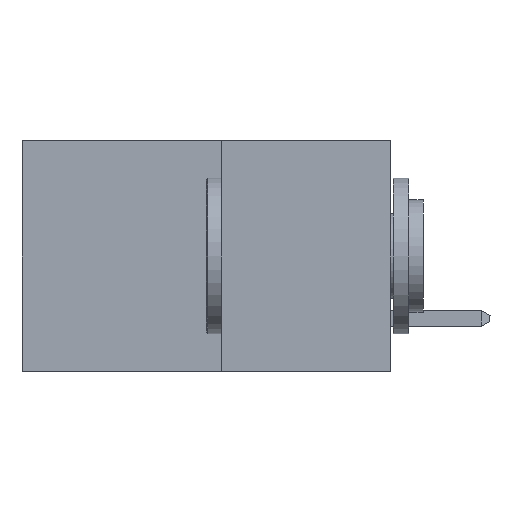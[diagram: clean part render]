
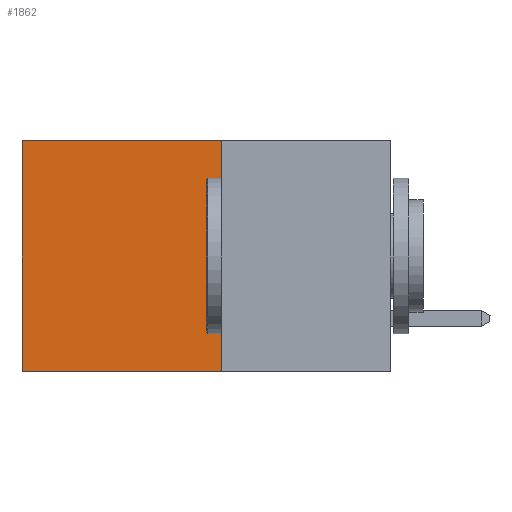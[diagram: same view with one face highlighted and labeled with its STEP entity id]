
A CAD part, left-side view. The second image highlights one B-rep face of the part: STEP entity #1862.
In plain terms, the highlighted planar face has unit normal (-1, 0, 0).
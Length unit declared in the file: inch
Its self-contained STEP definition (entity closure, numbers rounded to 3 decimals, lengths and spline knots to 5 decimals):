
#236 = VERTEX_POINT ( 'NONE', #5862 ) ;
#304 = EDGE_CURVE ( 'NONE', #2971, #236, #8479, .T. ) ;
#380 = VECTOR ( 'NONE', #4563, 39.37008 ) ;
#1190 = ORIENTED_EDGE ( 'NONE', *, *, #304, .T. ) ;
#1862 = ADVANCED_FACE ( 'NONE', ( #7123 ), #8314, .F. ) ;
#2348 = EDGE_LOOP ( 'NONE', ( #1190, #9143, #4047, #9275 ) ) ;
#2704 = DIRECTION ( 'NONE',  ( 0., 0., -1. ) ) ;
#2807 = CARTESIAN_POINT ( 'NONE',  ( 0.277, 0.59, -0.37 ) ) ;
#2971 = VERTEX_POINT ( 'NONE', #10305 ) ;
#3430 = CARTESIAN_POINT ( 'NONE',  ( 0.277, 0.27, 0. ) ) ;
#3478 = VECTOR ( 'NONE', #7276, 39.37008 ) ;
#3541 = VERTEX_POINT ( 'NONE', #11078 ) ;
#3650 = CARTESIAN_POINT ( 'NONE',  ( 0.277, 0.27, -0.37 ) ) ;
#4047 = ORIENTED_EDGE ( 'NONE', *, *, #7815, .F. ) ;
#4262 = LINE ( 'NONE', #6821, #6405 ) ;
#4563 = DIRECTION ( 'NONE',  ( 0., 1., 0. ) ) ;
#4685 = EDGE_CURVE ( 'NONE', #5410, #2971, #5909, .T. ) ;
#4697 = AXIS2_PLACEMENT_3D ( 'NONE', #8291, #5863, #6409 ) ;
#5410 = VERTEX_POINT ( 'NONE', #3430 ) ;
#5415 = LINE ( 'NONE', #3650, #380 ) ;
#5862 = CARTESIAN_POINT ( 'NONE',  ( 0.277, 0.59, -0.37 ) ) ;
#5863 = DIRECTION ( 'NONE',  ( 1., 0., 0. ) ) ;
#5909 = LINE ( 'NONE', #7553, #3478 ) ;
#6181 = VECTOR ( 'NONE', #2704, 39.37008 ) ;
#6405 = VECTOR ( 'NONE', #9379, 39.37008 ) ;
#6409 = DIRECTION ( 'NONE',  ( 0., 0., -1. ) ) ;
#6821 = CARTESIAN_POINT ( 'NONE',  ( 0.277, 0.27, -0.37 ) ) ;
#7123 = FACE_OUTER_BOUND ( 'NONE', #2348, .T. ) ;
#7276 = DIRECTION ( 'NONE',  ( 0., 1., 0. ) ) ;
#7553 = CARTESIAN_POINT ( 'NONE',  ( 0.277, 0.27, 0. ) ) ;
#7815 = EDGE_CURVE ( 'NONE', #5410, #3541, #4262, .T. ) ;
#8107 = EDGE_CURVE ( 'NONE', #3541, #236, #5415, .T. ) ;
#8291 = CARTESIAN_POINT ( 'NONE',  ( 0.277, 0.27, -0.37 ) ) ;
#8314 = PLANE ( 'NONE',  #4697 ) ;
#8479 = LINE ( 'NONE', #2807, #6181 ) ;
#9143 = ORIENTED_EDGE ( 'NONE', *, *, #8107, .F. ) ;
#9275 = ORIENTED_EDGE ( 'NONE', *, *, #4685, .T. ) ;
#9379 = DIRECTION ( 'NONE',  ( 0., 0., -1. ) ) ;
#10305 = CARTESIAN_POINT ( 'NONE',  ( 0.277, 0.59, 0. ) ) ;
#11078 = CARTESIAN_POINT ( 'NONE',  ( 0.277, 0.27, -0.37 ) ) ;
